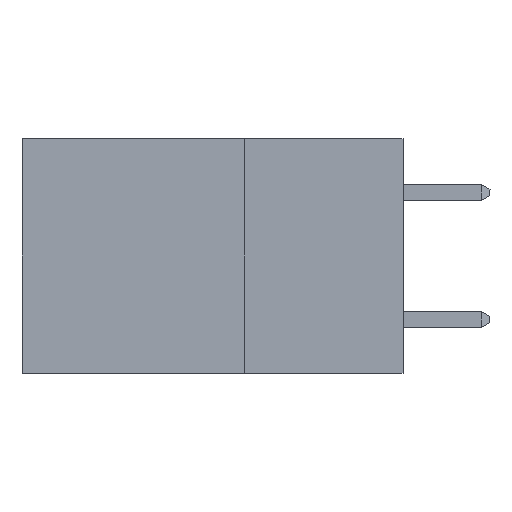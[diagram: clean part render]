
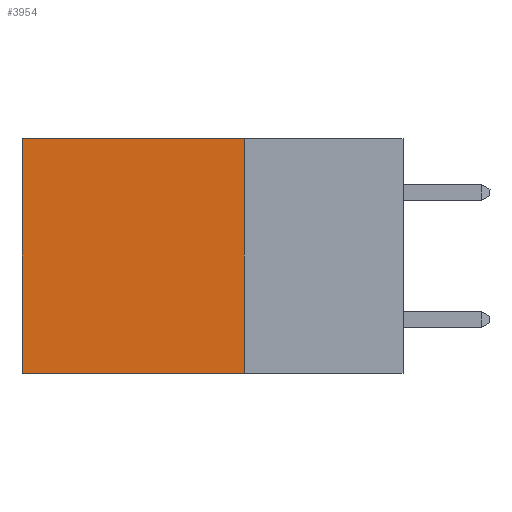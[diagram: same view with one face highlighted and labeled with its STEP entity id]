
A CAD part, left-side view. The second image highlights one B-rep face of the part: STEP entity #3954.
In plain terms, the highlighted planar face has unit normal (-1, 0, 0).
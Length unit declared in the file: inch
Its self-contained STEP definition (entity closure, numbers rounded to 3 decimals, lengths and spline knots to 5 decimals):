
#41 = ORIENTED_EDGE ( 'NONE', *, *, #10756, .T. ) ;
#106 = VERTEX_POINT ( 'NONE', #9410 ) ;
#843 = DIRECTION ( 'NONE',  ( 0., 0., -1. ) ) ;
#930 = ORIENTED_EDGE ( 'NONE', *, *, #10432, .T. ) ;
#1183 = DIRECTION ( 'NONE',  ( 0., 1., 0. ) ) ;
#1253 = EDGE_CURVE ( 'NONE', #4658, #106, #1416, .T. ) ;
#1416 = LINE ( 'NONE', #2023, #9705 ) ;
#1478 = DIRECTION ( 'NONE',  ( 0., 1., 0. ) ) ;
#2023 = CARTESIAN_POINT ( 'NONE',  ( 0.2875, 0.25, -0.37 ) ) ;
#2048 = DIRECTION ( 'NONE',  ( 0., 0., -1. ) ) ;
#3118 = VERTEX_POINT ( 'NONE', #11197 ) ;
#3319 = AXIS2_PLACEMENT_3D ( 'NONE', #11500, #6622, #12557 ) ;
#3911 = VECTOR ( 'NONE', #843, 39.37008 ) ;
#3954 = ADVANCED_FACE ( 'NONE', ( #5126 ), #7011, .F. ) ;
#4239 = VECTOR ( 'NONE', #1478, 39.37008 ) ;
#4572 = CARTESIAN_POINT ( 'NONE',  ( 0.2875, 0.25, -0.37 ) ) ;
#4658 = VERTEX_POINT ( 'NONE', #4572 ) ;
#5126 = FACE_OUTER_BOUND ( 'NONE', #7780, .T. ) ;
#5283 = EDGE_CURVE ( 'NONE', #3118, #4658, #10345, .T. ) ;
#6622 = DIRECTION ( 'NONE',  ( 1., 0., 0. ) ) ;
#7011 = PLANE ( 'NONE',  #3319 ) ;
#7560 = CARTESIAN_POINT ( 'NONE',  ( 0.2875, 0.6, 0. ) ) ;
#7699 = CARTESIAN_POINT ( 'NONE',  ( 0.2875, 0.6, 0. ) ) ;
#7780 = EDGE_LOOP ( 'NONE', ( #41, #12422, #10266, #930 ) ) ;
#8059 = CARTESIAN_POINT ( 'NONE',  ( 0.2875, 0.25, 0. ) ) ;
#8732 = LINE ( 'NONE', #7699, #3911 ) ;
#8888 = LINE ( 'NONE', #12189, #4239 ) ;
#9410 = CARTESIAN_POINT ( 'NONE',  ( 0.2875, 0.6, -0.37 ) ) ;
#9550 = VERTEX_POINT ( 'NONE', #7560 ) ;
#9705 = VECTOR ( 'NONE', #1183, 39.37008 ) ;
#10266 = ORIENTED_EDGE ( 'NONE', *, *, #5283, .F. ) ;
#10345 = LINE ( 'NONE', #8059, #11906 ) ;
#10432 = EDGE_CURVE ( 'NONE', #3118, #9550, #8888, .T. ) ;
#10756 = EDGE_CURVE ( 'NONE', #9550, #106, #8732, .T. ) ;
#11197 = CARTESIAN_POINT ( 'NONE',  ( 0.2875, 0.25, 0. ) ) ;
#11500 = CARTESIAN_POINT ( 'NONE',  ( 0.2875, 0.25, 0. ) ) ;
#11906 = VECTOR ( 'NONE', #2048, 39.37008 ) ;
#12189 = CARTESIAN_POINT ( 'NONE',  ( 0.2875, 0.25, 0. ) ) ;
#12422 = ORIENTED_EDGE ( 'NONE', *, *, #1253, .F. ) ;
#12557 = DIRECTION ( 'NONE',  ( 0., 0., -1. ) ) ;
